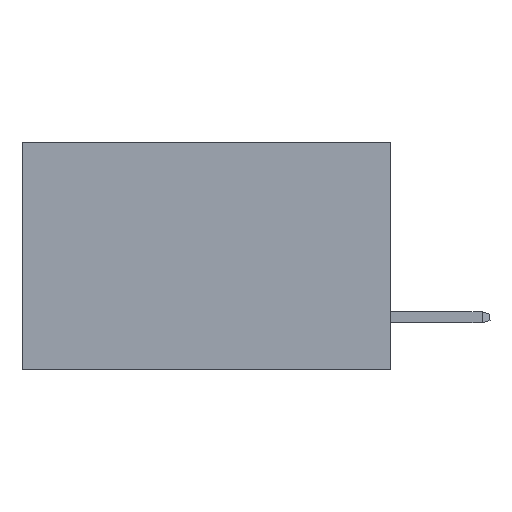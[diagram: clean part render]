
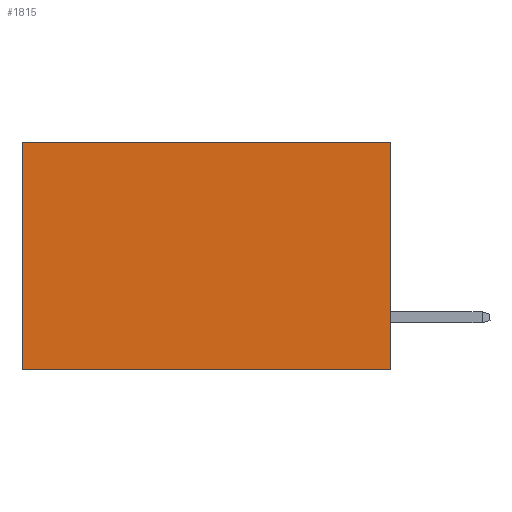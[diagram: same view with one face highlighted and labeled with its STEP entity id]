
A CAD part, left-side view. The second image highlights one B-rep face of the part: STEP entity #1815.
In plain terms, the highlighted planar face has unit normal (-1, 0, 0).
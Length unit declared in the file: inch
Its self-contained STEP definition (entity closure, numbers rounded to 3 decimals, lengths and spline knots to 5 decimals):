
#144 = ORIENTED_EDGE ( 'NONE', *, *, #4351, .T. ) ;
#192 = DIRECTION ( 'NONE',  ( 0., 1., 0. ) ) ;
#457 = VERTEX_POINT ( 'NONE', #11854 ) ;
#868 = ORIENTED_EDGE ( 'NONE', *, *, #3608, .F. ) ;
#1411 = CARTESIAN_POINT ( 'NONE',  ( 0.2875, 0., -0.37 ) ) ;
#1815 = ADVANCED_FACE ( 'NONE', ( #5588 ), #5295, .F. ) ;
#1933 = VECTOR ( 'NONE', #8152, 39.37008 ) ;
#2492 = DIRECTION ( 'NONE',  ( 1., 0., 0. ) ) ;
#2549 = CARTESIAN_POINT ( 'NONE',  ( 0.2875, 0.6, -0.37 ) ) ;
#2934 = EDGE_CURVE ( 'NONE', #11594, #11193, #4431, .T. ) ;
#3379 = CARTESIAN_POINT ( 'NONE',  ( 0.2875, 0., 0. ) ) ;
#3608 = EDGE_CURVE ( 'NONE', #457, #4761, #7151, .T. ) ;
#4351 = EDGE_CURVE ( 'NONE', #457, #11594, #11879, .T. ) ;
#4431 = LINE ( 'NONE', #10151, #9150 ) ;
#4543 = LINE ( 'NONE', #1411, #1933 ) ;
#4574 = VECTOR ( 'NONE', #6692, 39.37008 ) ;
#4761 = VERTEX_POINT ( 'NONE', #12043 ) ;
#4946 = VECTOR ( 'NONE', #192, 39.37008 ) ;
#5295 = PLANE ( 'NONE',  #8941 ) ;
#5429 = ORIENTED_EDGE ( 'NONE', *, *, #2934, .T. ) ;
#5560 = ORIENTED_EDGE ( 'NONE', *, *, #8320, .F. ) ;
#5588 = FACE_OUTER_BOUND ( 'NONE', #8646, .T. ) ;
#6142 = CARTESIAN_POINT ( 'NONE',  ( 0.2875, 0.6, 0. ) ) ;
#6692 = DIRECTION ( 'NONE',  ( 0., 0., -1. ) ) ;
#7151 = LINE ( 'NONE', #12238, #4574 ) ;
#8152 = DIRECTION ( 'NONE',  ( 0., 1., 0. ) ) ;
#8320 = EDGE_CURVE ( 'NONE', #4761, #11193, #4543, .T. ) ;
#8646 = EDGE_LOOP ( 'NONE', ( #5429, #5560, #868, #144 ) ) ;
#8941 = AXIS2_PLACEMENT_3D ( 'NONE', #3379, #2492, #10446 ) ;
#9150 = VECTOR ( 'NONE', #9390, 39.37008 ) ;
#9390 = DIRECTION ( 'NONE',  ( 0., 0., -1. ) ) ;
#10151 = CARTESIAN_POINT ( 'NONE',  ( 0.2875, 0.6, 0. ) ) ;
#10446 = DIRECTION ( 'NONE',  ( 0., 0., -1. ) ) ;
#11193 = VERTEX_POINT ( 'NONE', #2549 ) ;
#11594 = VERTEX_POINT ( 'NONE', #6142 ) ;
#11608 = CARTESIAN_POINT ( 'NONE',  ( 0.2875, 0., 0. ) ) ;
#11854 = CARTESIAN_POINT ( 'NONE',  ( 0.2875, 0., 0. ) ) ;
#11879 = LINE ( 'NONE', #11608, #4946 ) ;
#12043 = CARTESIAN_POINT ( 'NONE',  ( 0.2875, 0., -0.37 ) ) ;
#12238 = CARTESIAN_POINT ( 'NONE',  ( 0.2875, 0., 0. ) ) ;
